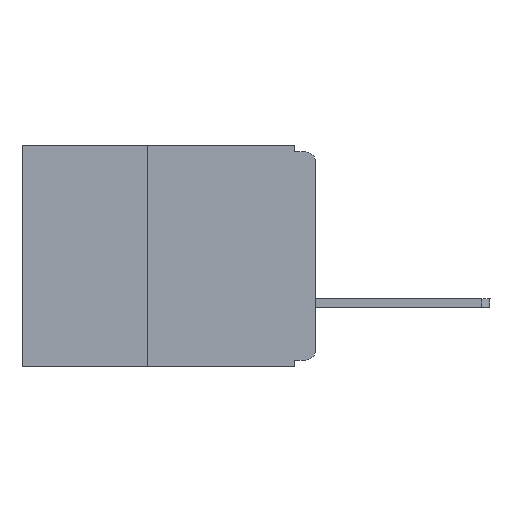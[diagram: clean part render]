
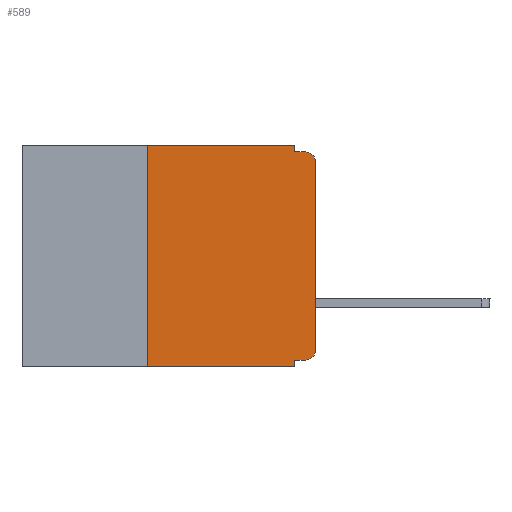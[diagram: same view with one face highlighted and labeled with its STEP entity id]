
A CAD part, left-side view. The second image highlights one B-rep face of the part: STEP entity #589.
In plain terms, the highlighted planar face has unit normal (-1, 0, 0).
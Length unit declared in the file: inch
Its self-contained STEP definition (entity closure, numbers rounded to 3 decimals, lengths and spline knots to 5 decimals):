
#7 = ORIENTED_EDGE ( 'NONE', *, *, #5955, .F. ) ;
#12 = VERTEX_POINT ( 'NONE', #3450 ) ;
#495 = DIRECTION ( 'NONE',  ( -1., 0., 0. ) ) ;
#589 = ADVANCED_FACE ( 'NONE', ( #6023 ), #8694, .F. ) ;
#1342 = CARTESIAN_POINT ( 'NONE',  ( 0., 0.015, -0.32 ) ) ;
#1535 = VECTOR ( 'NONE', #2817, 39.37008 ) ;
#1550 = LINE ( 'NONE', #4060, #5546 ) ;
#2231 = EDGE_CURVE ( 'NONE', #11413, #10069, #9642, .T. ) ;
#2817 = DIRECTION ( 'NONE',  ( 0., -1., 0. ) ) ;
#3254 = ORIENTED_EDGE ( 'NONE', *, *, #11966, .T. ) ;
#3404 = CARTESIAN_POINT ( 'NONE',  ( 0., 0.437, 0. ) ) ;
#3450 = CARTESIAN_POINT ( 'NONE',  ( 0., 0.25, -0.33 ) ) ;
#3561 = VECTOR ( 'NONE', #6217, 39.37008 ) ;
#3591 = DIRECTION ( 'NONE',  ( 0., 0., 1. ) ) ;
#3699 = DIRECTION ( 'NONE',  ( 0., -1., 0. ) ) ;
#3728 = EDGE_CURVE ( 'NONE', #3923, #8725, #1550, .T. ) ;
#3732 = CARTESIAN_POINT ( 'NONE',  ( 0., 0., 0. ) ) ;
#3873 = EDGE_CURVE ( 'NONE', #12, #10069, #9178, .T. ) ;
#3923 = VERTEX_POINT ( 'NONE', #8986 ) ;
#4014 = LINE ( 'NONE', #11092, #12483 ) ;
#4060 = CARTESIAN_POINT ( 'NONE',  ( 0., 0.031, 0. ) ) ;
#4192 = CARTESIAN_POINT ( 'NONE',  ( 0., 0.25, 0. ) ) ;
#4259 = VECTOR ( 'NONE', #13699, 39.37008 ) ;
#4271 = LINE ( 'NONE', #5258, #3561 ) ;
#4318 = DIRECTION ( 'NONE',  ( 0., 0., -1. ) ) ;
#4620 = CARTESIAN_POINT ( 'NONE',  ( 0., 0.015, -0.01 ) ) ;
#5208 = VERTEX_POINT ( 'NONE', #9217 ) ;
#5258 = CARTESIAN_POINT ( 'NONE',  ( 0., 0., -0.32 ) ) ;
#5350 = ORIENTED_EDGE ( 'NONE', *, *, #8609, .F. ) ;
#5399 = ORIENTED_EDGE ( 'NONE', *, *, #3873, .T. ) ;
#5546 = VECTOR ( 'NONE', #9590, 39.37008 ) ;
#5919 = CARTESIAN_POINT ( 'NONE',  ( 0., 0., -0.01 ) ) ;
#5955 = EDGE_CURVE ( 'NONE', #12288, #11413, #4271, .T. ) ;
#6015 = DIRECTION ( 'NONE',  ( 0., 0., -1. ) ) ;
#6023 = FACE_OUTER_BOUND ( 'NONE', #6193, .T. ) ;
#6092 = CARTESIAN_POINT ( 'NONE',  ( 0., 0.031, -0.33 ) ) ;
#6193 = EDGE_LOOP ( 'NONE', ( #3254, #12119, #6243, #8225, #13586, #5350, #5399, #7424, #7, #12687 ) ) ;
#6217 = DIRECTION ( 'NONE',  ( 0., 1., 0. ) ) ;
#6230 = VECTOR ( 'NONE', #12434, 39.37008 ) ;
#6243 = ORIENTED_EDGE ( 'NONE', *, *, #8799, .F. ) ;
#6426 = AXIS2_PLACEMENT_3D ( 'NONE', #3404, #9834, #4318 ) ;
#6608 = VERTEX_POINT ( 'NONE', #12541 ) ;
#6914 = CARTESIAN_POINT ( 'NONE',  ( 0., 0.437, -0.33 ) ) ;
#7081 = LINE ( 'NONE', #3732, #10324 ) ;
#7424 = ORIENTED_EDGE ( 'NONE', *, *, #2231, .F. ) ;
#7552 = EDGE_CURVE ( 'NONE', #6608, #12084, #8230, .T. ) ;
#8225 = ORIENTED_EDGE ( 'NONE', *, *, #3728, .F. ) ;
#8230 = CIRCLE ( 'NONE', #13043, 0.015 ) ;
#8359 = CARTESIAN_POINT ( 'NONE',  ( 0., 0.015, -0.305 ) ) ;
#8609 = EDGE_CURVE ( 'NONE', #12, #12860, #4014, .T. ) ;
#8694 = PLANE ( 'NONE',  #6426 ) ;
#8725 = VERTEX_POINT ( 'NONE', #12437 ) ;
#8799 = EDGE_CURVE ( 'NONE', #8725, #12084, #9208, .T. ) ;
#8986 = CARTESIAN_POINT ( 'NONE',  ( 0., 0.031, 0. ) ) ;
#9178 = LINE ( 'NONE', #6914, #6230 ) ;
#9208 = LINE ( 'NONE', #5919, #13536 ) ;
#9217 = CARTESIAN_POINT ( 'NONE',  ( 0., 0., -0.305 ) ) ;
#9590 = DIRECTION ( 'NONE',  ( 0., 0., -1. ) ) ;
#9642 = LINE ( 'NONE', #6092, #4259 ) ;
#9834 = DIRECTION ( 'NONE',  ( 1., 0., 0. ) ) ;
#10069 = VERTEX_POINT ( 'NONE', #10998 ) ;
#10324 = VECTOR ( 'NONE', #3591, 39.37008 ) ;
#10400 = CARTESIAN_POINT ( 'NONE',  ( 0., 0.437, 0. ) ) ;
#10481 = DIRECTION ( 'NONE',  ( 0., 0., -1. ) ) ;
#10685 = CARTESIAN_POINT ( 'NONE',  ( 0., 0.031, -0.32 ) ) ;
#10902 = EDGE_CURVE ( 'NONE', #12860, #3923, #14181, .T. ) ;
#10998 = CARTESIAN_POINT ( 'NONE',  ( 0., 0.031, -0.33 ) ) ;
#11092 = CARTESIAN_POINT ( 'NONE',  ( 0., 0.25, -0.33 ) ) ;
#11413 = VERTEX_POINT ( 'NONE', #10685 ) ;
#11527 = CARTESIAN_POINT ( 'NONE',  ( 0., 0.015, -0.025 ) ) ;
#11966 = EDGE_CURVE ( 'NONE', #5208, #6608, #7081, .T. ) ;
#12084 = VERTEX_POINT ( 'NONE', #4620 ) ;
#12119 = ORIENTED_EDGE ( 'NONE', *, *, #7552, .T. ) ;
#12288 = VERTEX_POINT ( 'NONE', #1342 ) ;
#12336 = EDGE_CURVE ( 'NONE', #12288, #5208, #12927, .T. ) ;
#12434 = DIRECTION ( 'NONE',  ( 0., -1., 0. ) ) ;
#12437 = CARTESIAN_POINT ( 'NONE',  ( 0., 0.031, -0.01 ) ) ;
#12483 = VECTOR ( 'NONE', #13323, 39.37008 ) ;
#12541 = CARTESIAN_POINT ( 'NONE',  ( 0., 0., -0.025 ) ) ;
#12580 = DIRECTION ( 'NONE',  ( -1., 0., 0. ) ) ;
#12687 = ORIENTED_EDGE ( 'NONE', *, *, #12336, .T. ) ;
#12860 = VERTEX_POINT ( 'NONE', #4192 ) ;
#12927 = CIRCLE ( 'NONE', #13357, 0.015 ) ;
#13043 = AXIS2_PLACEMENT_3D ( 'NONE', #11527, #12580, #6015 ) ;
#13323 = DIRECTION ( 'NONE',  ( 0., 0., 1. ) ) ;
#13357 = AXIS2_PLACEMENT_3D ( 'NONE', #8359, #495, #10481 ) ;
#13536 = VECTOR ( 'NONE', #3699, 39.37008 ) ;
#13586 = ORIENTED_EDGE ( 'NONE', *, *, #10902, .F. ) ;
#13699 = DIRECTION ( 'NONE',  ( 0., 0., -1. ) ) ;
#14181 = LINE ( 'NONE', #10400, #1535 ) ;
